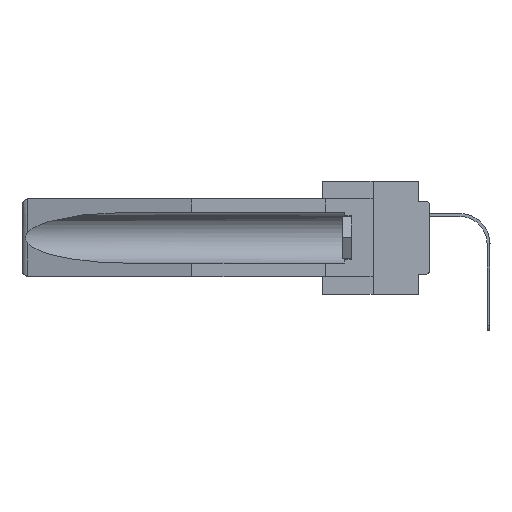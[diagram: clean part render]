
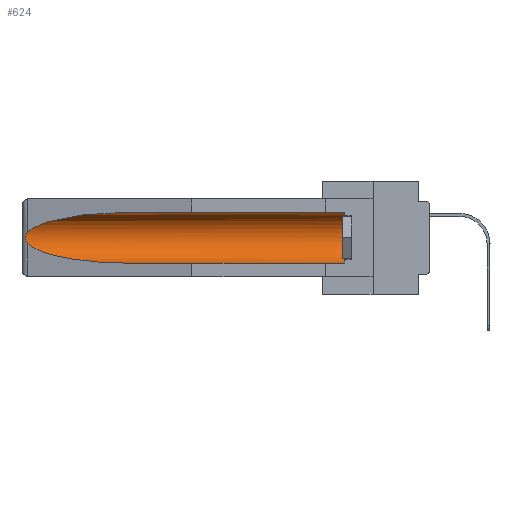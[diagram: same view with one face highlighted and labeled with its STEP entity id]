
A CAD part, left-side view. The second image highlights one B-rep face of the part: STEP entity #624.
In plain terms, the highlighted cylindrical face has radius 2.857 mm (diameter 5.715 mm), a partial arc.
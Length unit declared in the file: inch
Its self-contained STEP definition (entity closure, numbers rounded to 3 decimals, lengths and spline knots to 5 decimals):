
#60 = CARTESIAN_POINT ( 'NONE',  ( 0.26655, 1.53094, -0.18657 ) ) ;
#374 = CARTESIAN_POINT ( 'NONE',  ( 0.2673, 1.53269, -0.17917 ) ) ;
#624 = ADVANCED_FACE ( 'NONE', ( #26684 ), #31660, .F. ) ;
#1243 = EDGE_CURVE ( 'NONE', #22158, #13676, #22833, .T. ) ;
#2331 = CARTESIAN_POINT ( 'NONE',  ( 0.155, 1.07973, -0.284 ) ) ;
#2335 = CARTESIAN_POINT ( 'NONE',  ( 0.155, 1.07973, -0.059 ) ) ;
#2511 = CARTESIAN_POINT ( 'NONE',  ( 0.2673, 1.5327, -0.16383 ) ) ;
#2744 = DIRECTION ( 'NONE',  ( 0., 1., 0. ) ) ;
#3551 = VECTOR ( 'NONE', #20088, 39.37008 ) ;
#4978 = CARTESIAN_POINT ( 'NONE',  ( 0.26537, 1.52718, -0.14972 ) ) ;
#5024 = EDGE_CURVE ( 'NONE', #6893, #15481, #22735, .T. ) ;
#5107 = DIRECTION ( 'NONE',  ( 0., 0., 1. ) ) ;
#6893 = VERTEX_POINT ( 'NONE', #27025 ) ;
#7814 = ORIENTED_EDGE ( 'NONE', *, *, #10646, .T. ) ;
#7886 = ORIENTED_EDGE ( 'NONE', *, *, #1243, .F. ) ;
#8978 = CARTESIAN_POINT ( 'NONE',  ( 0.155, -0.30754, -0.1715 ) ) ;
#9013 = ORIENTED_EDGE ( 'NONE', *, *, #10257, .T. ) ;
#9628 = DIRECTION ( 'NONE',  ( 0., 1., 0. ) ) ;
#10089 =( BOUNDED_CURVE ( )  B_SPLINE_CURVE ( 3, ( #2335, #12286, #22237, #19747 ),
 .UNSPECIFIED., .F., .F. ) 
 B_SPLINE_CURVE_WITH_KNOTS ( ( 4, 4 ),
 ( 4.71239, 6.08839 ),
 .UNSPECIFIED. ) 
 CURVE ( )  GEOMETRIC_REPRESENTATION_ITEM ( )  RATIONAL_B_SPLINE_CURVE ( ( 1., 0.848, 0.848, 1. ) ) 
 REPRESENTATION_ITEM ( '' )  );
#10140 = CARTESIAN_POINT ( 'NONE',  ( 0.26537, 1.52718, -0.19328 ) ) ;
#10257 = EDGE_CURVE ( 'NONE', #19828, #12631, #26754, .T. ) ;
#10478 =( BOUNDED_CURVE ( )  B_SPLINE_CURVE ( 3, ( #12616, #15432, #14777, #2331 ),
 .UNSPECIFIED., .F., .F. ) 
 B_SPLINE_CURVE_WITH_KNOTS ( ( 4, 4 ),
 ( 0.1948, 1.5708 ),
 .UNSPECIFIED. ) 
 CURVE ( )  GEOMETRIC_REPRESENTATION_ITEM ( )  RATIONAL_B_SPLINE_CURVE ( ( 1., 0.848, 0.848, 1. ) ) 
 REPRESENTATION_ITEM ( '' )  );
#10646 = EDGE_CURVE ( 'NONE', #22158, #6893, #32294, .T. ) ;
#10846 = AXIS2_PLACEMENT_3D ( 'NONE', #8978, #9628, #19089 ) ;
#10985 = ORIENTED_EDGE ( 'NONE', *, *, #22597, .T. ) ;
#11966 = CARTESIAN_POINT ( 'NONE',  ( 0.155, -0.30754, -0.059 ) ) ;
#12286 = CARTESIAN_POINT ( 'NONE',  ( 0.21114, 1.30732, -0.059 ) ) ;
#12616 = CARTESIAN_POINT ( 'NONE',  ( 0.26537, 1.52718, -0.19328 ) ) ;
#12631 = VERTEX_POINT ( 'NONE', #24277 ) ;
#12721 = ORIENTED_EDGE ( 'NONE', *, *, #5024, .T. ) ;
#13106 = CARTESIAN_POINT ( 'NONE',  ( 0.26597, 1.5296, -0.19026 ) ) ;
#13167 = EDGE_CURVE ( 'NONE', #15481, #19828, #10089, .T. ) ;
#13676 = VERTEX_POINT ( 'NONE', #18516 ) ;
#14777 = CARTESIAN_POINT ( 'NONE',  ( 0.21114, 1.30732, -0.284 ) ) ;
#15432 = CARTESIAN_POINT ( 'NONE',  ( 0.25451, 1.48313, -0.24835 ) ) ;
#15481 = VERTEX_POINT ( 'NONE', #31086 ) ;
#17397 = CARTESIAN_POINT ( 'NONE',  ( 0.155, 0.126, -0.1715 ) ) ;
#17496 = CARTESIAN_POINT ( 'NONE',  ( 0.155, 0.126, -0.284 ) ) ;
#17594 = CARTESIAN_POINT ( 'NONE',  ( 0.26654, 1.53092, -0.15636 ) ) ;
#18516 = CARTESIAN_POINT ( 'NONE',  ( 0.155, 1.07973, -0.284 ) ) ;
#18820 = VECTOR ( 'NONE', #2744, 39.37008 ) ;
#19089 = DIRECTION ( 'NONE',  ( 0., 0., 1. ) ) ;
#19623 = AXIS2_PLACEMENT_3D ( 'NONE', #17397, #25148, #5107 ) ;
#19747 = CARTESIAN_POINT ( 'NONE',  ( 0.26537, 1.52718, -0.14972 ) ) ;
#19828 = VERTEX_POINT ( 'NONE', #20992 ) ;
#20088 = DIRECTION ( 'NONE',  ( 0., 1., 0. ) ) ;
#20992 = CARTESIAN_POINT ( 'NONE',  ( 0.26537, 1.52718, -0.14972 ) ) ;
#22158 = VERTEX_POINT ( 'NONE', #17496 ) ;
#22237 = CARTESIAN_POINT ( 'NONE',  ( 0.25451, 1.48313, -0.09465 ) ) ;
#22597 = EDGE_CURVE ( 'NONE', #12631, #13676, #10478, .T. ) ;
#22665 = CARTESIAN_POINT ( 'NONE',  ( 0.155, -0.30754, -0.284 ) ) ;
#22735 = LINE ( 'NONE', #11966, #3551 ) ;
#22833 = LINE ( 'NONE', #22665, #18820 ) ;
#22889 = CARTESIAN_POINT ( 'NONE',  ( 0.26597, 1.52961, -0.15275 ) ) ;
#24277 = CARTESIAN_POINT ( 'NONE',  ( 0.26537, 1.52718, -0.19328 ) ) ;
#25148 = DIRECTION ( 'NONE',  ( 0., -1., 0. ) ) ;
#26684 = FACE_OUTER_BOUND ( 'NONE', #30354, .T. ) ;
#26754 = B_SPLINE_CURVE_WITH_KNOTS ( 'NONE', 3,
 ( #4978, #22889, #17594, #2511, #28165, #27679, #374, #60, #13106, #10140 ),
 .UNSPECIFIED., .F., .F.,
 ( 4, 2, 2, 2, 4 ),
 ( 0., 0.00029, 0.00058, 0.00087, 0.00117 ),
 .UNSPECIFIED. ) ;
#27025 = CARTESIAN_POINT ( 'NONE',  ( 0.155, 0.126, -0.059 ) ) ;
#27679 = CARTESIAN_POINT ( 'NONE',  ( 0.2675, 1.53308, -0.17534 ) ) ;
#28165 = CARTESIAN_POINT ( 'NONE',  ( 0.2675, 1.53308, -0.16763 ) ) ;
#30354 = EDGE_LOOP ( 'NONE', ( #32070, #9013, #10985, #7886, #7814, #12721 ) ) ;
#31086 = CARTESIAN_POINT ( 'NONE',  ( 0.155, 1.07973, -0.059 ) ) ;
#31660 = CYLINDRICAL_SURFACE ( 'NONE', #10846, 0.1125 ) ;
#32070 = ORIENTED_EDGE ( 'NONE', *, *, #13167, .T. ) ;
#32294 = CIRCLE ( 'NONE', #19623, 0.1125 ) ;
